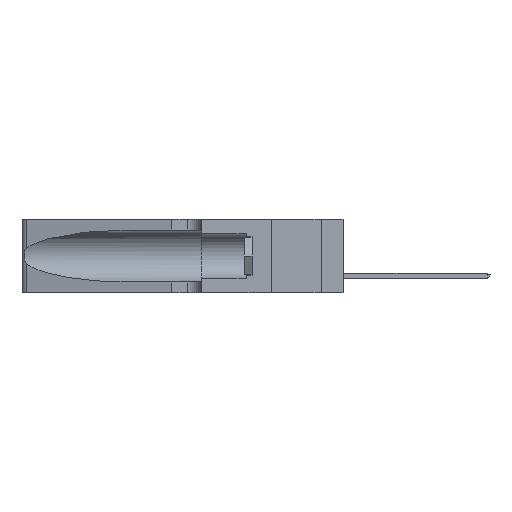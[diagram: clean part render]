
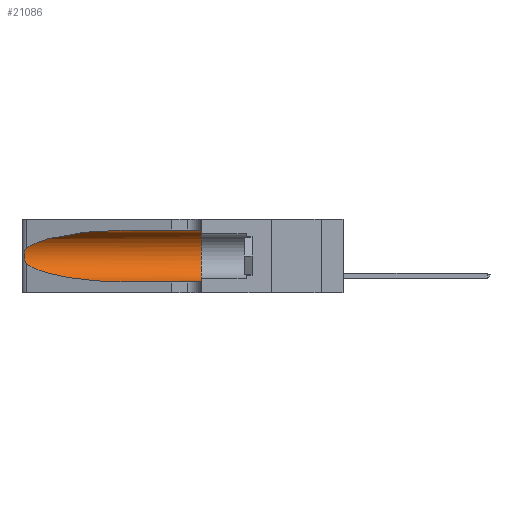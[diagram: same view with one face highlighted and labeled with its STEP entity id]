
A CAD part, left-side view. The second image highlights one B-rep face of the part: STEP entity #21086.
In plain terms, the highlighted cylindrical face has radius 3.308 mm (diameter 6.617 mm), a partial arc.
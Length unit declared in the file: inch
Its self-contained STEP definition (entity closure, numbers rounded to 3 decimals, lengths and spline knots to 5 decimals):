
#361 = CARTESIAN_POINT ( 'NONE',  ( 0.2373, 1.15595, 0.28018 ) ) ;
#665 =( BOUNDED_CURVE ( )  B_SPLINE_CURVE ( 3, ( #21325, #15347, #361, #13780 ),
 .UNSPECIFIED., .F., .F. ) 
 B_SPLINE_CURVE_WITH_KNOTS ( ( 4, 4 ),
 ( 1.5708, 2.84003 ),
 .UNSPECIFIED. ) 
 CURVE ( )  GEOMETRIC_REPRESENTATION_ITEM ( )  RATIONAL_B_SPLINE_CURVE ( ( 1., 0.87, 0.87, 1. ) ) 
 REPRESENTATION_ITEM ( '' )  );
#1275 = CARTESIAN_POINT ( 'NONE',  ( 0.26017, 1.23833, 0.17102 ) ) ;
#1473 = CARTESIAN_POINT ( 'NONE',  ( 0.1305, 0.35, 0.185 ) ) ;
#1484 = VERTEX_POINT ( 'NONE', #14015 ) ;
#1530 = CARTESIAN_POINT ( 'NONE',  ( 0.26018, 1.23835, 0.19895 ) ) ;
#1538 = VERTEX_POINT ( 'NONE', #20066 ) ;
#3417 = CARTESIAN_POINT ( 'NONE',  ( 0.26075, 1.23896, 0.178 ) ) ;
#3501 = CARTESIAN_POINT ( 'NONE',  ( 0.1305, 0.72297, 0.05475 ) ) ;
#3502 = CARTESIAN_POINT ( 'NONE',  ( 0.25487, 1.22718, 0.14631 ) ) ;
#5051 = CARTESIAN_POINT ( 'NONE',  ( 0.25555, 1.22994, 0.2215 ) ) ;
#5081 = VERTEX_POINT ( 'NONE', #14125 ) ;
#5450 = CARTESIAN_POINT ( 'NONE',  ( 0.1305, 1.61858, 0.185 ) ) ;
#5487 = DIRECTION ( 'NONE',  ( 0., 1., 0. ) ) ;
#5968 = DIRECTION ( 'NONE',  ( 0., -1., 0. ) ) ;
#6130 = CARTESIAN_POINT ( 'NONE',  ( 0.1305, 1.61858, 0.31525 ) ) ;
#6560 = CARTESIAN_POINT ( 'NONE',  ( 0.25487, 1.22718, 0.14631 ) ) ;
#7035 = EDGE_LOOP ( 'NONE', ( #23925, #23493, #23292, #20402, #14681, #17584 ) ) ;
#7410 = DIRECTION ( 'NONE',  ( 0., 0., -1. ) ) ;
#8001 = CIRCLE ( 'NONE', #14971, 0.13025 ) ;
#8299 = CARTESIAN_POINT ( 'NONE',  ( 0.25487, 1.22718, 0.22369 ) ) ;
#8443 = CYLINDRICAL_SURFACE ( 'NONE', #20019, 0.13025 ) ;
#8841 = CARTESIAN_POINT ( 'NONE',  ( 0.25854, 1.2359, 0.20912 ) ) ;
#9021 = CARTESIAN_POINT ( 'NONE',  ( 0.18966, 0.96281, 0.05475 ) ) ;
#9213 = VERTEX_POINT ( 'NONE', #24097 ) ;
#9440 = EDGE_CURVE ( 'NONE', #14888, #12802, #22608, .T. ) ;
#11672 = LINE ( 'NONE', #6130, #20520 ) ;
#12299 = EDGE_CURVE ( 'NONE', #1484, #9213, #20845, .T. ) ;
#12658 = CARTESIAN_POINT ( 'NONE',  ( 0.25555, 1.22993, 0.14849 ) ) ;
#12778 = DIRECTION ( 'NONE',  ( 0., -1., 0. ) ) ;
#12802 = VERTEX_POINT ( 'NONE', #20322 ) ;
#13109 = DIRECTION ( 'NONE',  ( 0., 0., 1. ) ) ;
#13508 = FACE_OUTER_BOUND ( 'NONE', #7035, .T. ) ;
#13780 = CARTESIAN_POINT ( 'NONE',  ( 0.25487, 1.22718, 0.22369 ) ) ;
#13895 =( BOUNDED_CURVE ( )  B_SPLINE_CURVE ( 3, ( #6560, #14564, #9021, #3501 ),
 .UNSPECIFIED., .F., .T. ) 
 B_SPLINE_CURVE_WITH_KNOTS ( ( 4, 4 ),
 ( 3.44316, 4.71239 ),
 .UNSPECIFIED. ) 
 CURVE ( )  GEOMETRIC_REPRESENTATION_ITEM ( )  RATIONAL_B_SPLINE_CURVE ( ( 1., 0.87, 0.87, 1. ) ) 
 REPRESENTATION_ITEM ( '' )  );
#14015 = CARTESIAN_POINT ( 'NONE',  ( 0.1305, 0.72297, 0.05475 ) ) ;
#14125 = CARTESIAN_POINT ( 'NONE',  ( 0.1305, 0.35, 0.31525 ) ) ;
#14478 = CARTESIAN_POINT ( 'NONE',  ( 0.25639, 1.23186, 0.15144 ) ) ;
#14513 = CARTESIAN_POINT ( 'NONE',  ( 0.1305, 1.61858, 0.05475 ) ) ;
#14564 = CARTESIAN_POINT ( 'NONE',  ( 0.2373, 1.15595, 0.08982 ) ) ;
#14637 = DIRECTION ( 'NONE',  ( 0., -1., 0. ) ) ;
#14681 = ORIENTED_EDGE ( 'NONE', *, *, #17898, .F. ) ;
#14888 = VERTEX_POINT ( 'NONE', #8299 ) ;
#14971 = AXIS2_PLACEMENT_3D ( 'NONE', #1473, #5487, #13109 ) ;
#15347 = CARTESIAN_POINT ( 'NONE',  ( 0.18966, 0.96281, 0.31525 ) ) ;
#16343 = EDGE_CURVE ( 'NONE', #1538, #5081, #11672, .T. ) ;
#16352 = CARTESIAN_POINT ( 'NONE',  ( 0.25639, 1.23184, 0.21858 ) ) ;
#16603 = CARTESIAN_POINT ( 'NONE',  ( 0.25787, 1.23484, 0.2124 ) ) ;
#16812 = EDGE_CURVE ( 'NONE', #12802, #1484, #13895, .T. ) ;
#17520 = EDGE_CURVE ( 'NONE', #1538, #14888, #665, .T. ) ;
#17584 = ORIENTED_EDGE ( 'NONE', *, *, #16343, .F. ) ;
#17898 = EDGE_CURVE ( 'NONE', #5081, #9213, #8001, .T. ) ;
#18235 = CARTESIAN_POINT ( 'NONE',  ( 0.26075, 1.23896, 0.19203 ) ) ;
#20019 = AXIS2_PLACEMENT_3D ( 'NONE', #5450, #14637, #7410 ) ;
#20066 = CARTESIAN_POINT ( 'NONE',  ( 0.1305, 0.72297, 0.31525 ) ) ;
#20322 = CARTESIAN_POINT ( 'NONE',  ( 0.25487, 1.22718, 0.14631 ) ) ;
#20402 = ORIENTED_EDGE ( 'NONE', *, *, #12299, .T. ) ;
#20520 = VECTOR ( 'NONE', #5968, 39.37008 ) ;
#20845 = LINE ( 'NONE', #14513, #21721 ) ;
#21086 = ADVANCED_FACE ( 'NONE', ( #13508 ), #8443, .F. ) ;
#21325 = CARTESIAN_POINT ( 'NONE',  ( 0.1305, 0.72297, 0.31525 ) ) ;
#21721 = VECTOR ( 'NONE', #12778, 39.37008 ) ;
#22014 = CARTESIAN_POINT ( 'NONE',  ( 0.25789, 1.23486, 0.15765 ) ) ;
#22608 = B_SPLINE_CURVE_WITH_KNOTS ( 'NONE', 3,
 ( #24079, #5051, #16352, #16603, #8841, #1530, #18235, #3417, #1275, #24248, #22014, #14478, #12658, #3502 ),
 .UNSPECIFIED., .F., .F.,
 ( 4, 2, 2, 2, 2, 2, 4 ),
 ( 0., 0.00027, 0.00053, 0.00107, 0.0016, 0.00187, 0.00214 ),
 .UNSPECIFIED. ) ;
#23292 = ORIENTED_EDGE ( 'NONE', *, *, #16812, .T. ) ;
#23493 = ORIENTED_EDGE ( 'NONE', *, *, #9440, .T. ) ;
#23925 = ORIENTED_EDGE ( 'NONE', *, *, #17520, .T. ) ;
#24079 = CARTESIAN_POINT ( 'NONE',  ( 0.25487, 1.22718, 0.22369 ) ) ;
#24097 = CARTESIAN_POINT ( 'NONE',  ( 0.1305, 0.35, 0.05475 ) ) ;
#24248 = CARTESIAN_POINT ( 'NONE',  ( 0.25856, 1.23593, 0.16098 ) ) ;
